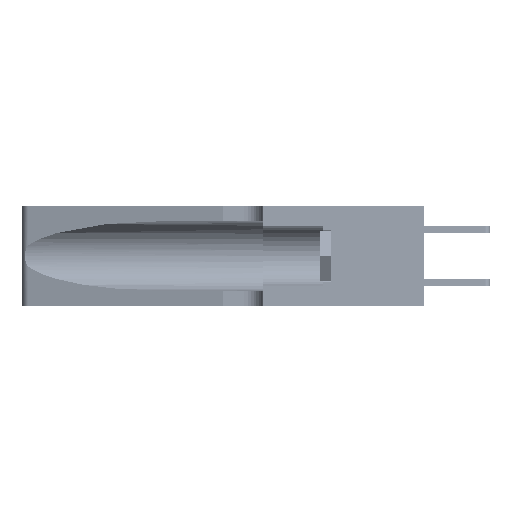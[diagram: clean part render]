
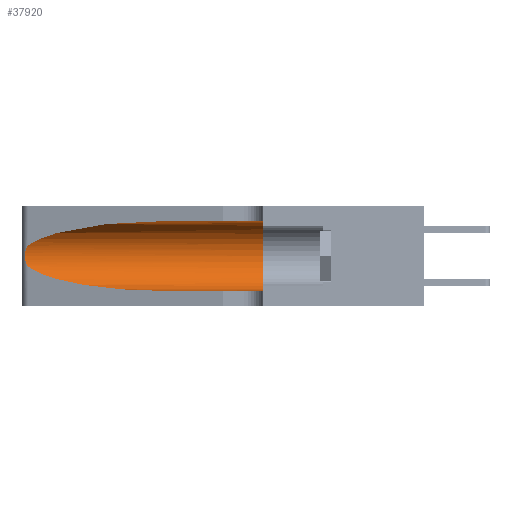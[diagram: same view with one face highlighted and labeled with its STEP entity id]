
A CAD part, left-side view. The second image highlights one B-rep face of the part: STEP entity #37920.
In plain terms, the highlighted cylindrical face has radius 3.308 mm (diameter 6.617 mm), a partial arc.
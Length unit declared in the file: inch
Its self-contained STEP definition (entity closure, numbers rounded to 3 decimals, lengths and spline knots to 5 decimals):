
#513 = CARTESIAN_POINT ( 'NONE',  ( 0.1305, 0.35, 0.185 ) ) ;
#750 = CIRCLE ( 'NONE', #49949, 0.13025 ) ;
#852 = VERTEX_POINT ( 'NONE', #14335 ) ;
#1556 =( BOUNDED_CURVE ( )  B_SPLINE_CURVE ( 3, ( #27196, #48484, #35395, #31410 ),
 .UNSPECIFIED., .F., .T. ) 
 B_SPLINE_CURVE_WITH_KNOTS ( ( 4, 4 ),
 ( 3.44316, 4.71239 ),
 .UNSPECIFIED. ) 
 CURVE ( )  GEOMETRIC_REPRESENTATION_ITEM ( )  RATIONAL_B_SPLINE_CURVE ( ( 1., 0.87, 0.87, 1. ) ) 
 REPRESENTATION_ITEM ( '' )  );
#1762 = CARTESIAN_POINT ( 'NONE',  ( 0.1305, 1.61858, 0.31525 ) ) ;
#3126 = CARTESIAN_POINT ( 'NONE',  ( 0.25555, 1.22994, 0.2215 ) ) ;
#3614 = ORIENTED_EDGE ( 'NONE', *, *, #16520, .F. ) ;
#4356 = DIRECTION ( 'NONE',  ( 0., 0., 1. ) ) ;
#5563 = CARTESIAN_POINT ( 'NONE',  ( 0.1305, 1.61858, 0.185 ) ) ;
#5946 = EDGE_LOOP ( 'NONE', ( #40991, #8715, #35002, #17758, #3614, #28600 ) ) ;
#7328 = CARTESIAN_POINT ( 'NONE',  ( 0.25856, 1.23593, 0.16098 ) ) ;
#8598 = VECTOR ( 'NONE', #21838, 39.37008 ) ;
#8715 = ORIENTED_EDGE ( 'NONE', *, *, #25585, .T. ) ;
#8809 = VERTEX_POINT ( 'NONE', #23151 ) ;
#9254 = DIRECTION ( 'NONE',  ( 0., 1., 0. ) ) ;
#10370 = EDGE_CURVE ( 'NONE', #8809, #38213, #12189, .T. ) ;
#10957 = CARTESIAN_POINT ( 'NONE',  ( 0.25487, 1.22718, 0.22369 ) ) ;
#11316 = CARTESIAN_POINT ( 'NONE',  ( 0.25555, 1.22993, 0.14849 ) ) ;
#12012 = CARTESIAN_POINT ( 'NONE',  ( 0.25487, 1.22718, 0.14631 ) ) ;
#12189 = LINE ( 'NONE', #1762, #20646 ) ;
#13992 = VERTEX_POINT ( 'NONE', #45386 ) ;
#14335 = CARTESIAN_POINT ( 'NONE',  ( 0.25487, 1.22718, 0.22369 ) ) ;
#14956 = CARTESIAN_POINT ( 'NONE',  ( 0.25639, 1.23186, 0.15144 ) ) ;
#15243 =( BOUNDED_CURVE ( )  B_SPLINE_CURVE ( 3, ( #47153, #22226, #26943, #43481 ),
 .UNSPECIFIED., .F., .F. ) 
 B_SPLINE_CURVE_WITH_KNOTS ( ( 4, 4 ),
 ( 1.5708, 2.84003 ),
 .UNSPECIFIED. ) 
 CURVE ( )  GEOMETRIC_REPRESENTATION_ITEM ( )  RATIONAL_B_SPLINE_CURVE ( ( 1., 0.87, 0.87, 1. ) ) 
 REPRESENTATION_ITEM ( '' )  );
#15687 = CARTESIAN_POINT ( 'NONE',  ( 0.25487, 1.22718, 0.14631 ) ) ;
#16520 = EDGE_CURVE ( 'NONE', #38213, #19927, #750, .T. ) ;
#17758 = ORIENTED_EDGE ( 'NONE', *, *, #53254, .T. ) ;
#18133 = VERTEX_POINT ( 'NONE', #12012 ) ;
#19146 = CARTESIAN_POINT ( 'NONE',  ( 0.25639, 1.23184, 0.21858 ) ) ;
#19323 = CARTESIAN_POINT ( 'NONE',  ( 0.26018, 1.23835, 0.19895 ) ) ;
#19927 = VERTEX_POINT ( 'NONE', #27743 ) ;
#20646 = VECTOR ( 'NONE', #52000, 39.37008 ) ;
#21592 = DIRECTION ( 'NONE',  ( 0., 0., -1. ) ) ;
#21838 = DIRECTION ( 'NONE',  ( 0., -1., 0. ) ) ;
#22226 = CARTESIAN_POINT ( 'NONE',  ( 0.18966, 0.96281, 0.31525 ) ) ;
#22706 = FACE_OUTER_BOUND ( 'NONE', #5946, .T. ) ;
#23151 = CARTESIAN_POINT ( 'NONE',  ( 0.1305, 0.72297, 0.31525 ) ) ;
#23886 = CARTESIAN_POINT ( 'NONE',  ( 0.26017, 1.23833, 0.17102 ) ) ;
#24083 = CARTESIAN_POINT ( 'NONE',  ( 0.26075, 1.23896, 0.178 ) ) ;
#25585 = EDGE_CURVE ( 'NONE', #852, #18133, #35574, .T. ) ;
#26383 = CARTESIAN_POINT ( 'NONE',  ( 0.1305, 1.61858, 0.05475 ) ) ;
#26943 = CARTESIAN_POINT ( 'NONE',  ( 0.2373, 1.15595, 0.28018 ) ) ;
#27196 = CARTESIAN_POINT ( 'NONE',  ( 0.25487, 1.22718, 0.14631 ) ) ;
#27743 = CARTESIAN_POINT ( 'NONE',  ( 0.1305, 0.35, 0.05475 ) ) ;
#28247 = CARTESIAN_POINT ( 'NONE',  ( 0.25854, 1.2359, 0.20912 ) ) ;
#28600 = ORIENTED_EDGE ( 'NONE', *, *, #10370, .F. ) ;
#31410 = CARTESIAN_POINT ( 'NONE',  ( 0.1305, 0.72297, 0.05475 ) ) ;
#31916 = CARTESIAN_POINT ( 'NONE',  ( 0.26075, 1.23896, 0.19203 ) ) ;
#33375 = EDGE_CURVE ( 'NONE', #8809, #852, #15243, .T. ) ;
#33853 = AXIS2_PLACEMENT_3D ( 'NONE', #5563, #33961, #21592 ) ;
#33961 = DIRECTION ( 'NONE',  ( 0., -1., 0. ) ) ;
#35002 = ORIENTED_EDGE ( 'NONE', *, *, #40027, .T. ) ;
#35395 = CARTESIAN_POINT ( 'NONE',  ( 0.18966, 0.96281, 0.05475 ) ) ;
#35574 = B_SPLINE_CURVE_WITH_KNOTS ( 'NONE', 3,
 ( #10957, #3126, #19146, #35889, #28247, #19323, #31916, #24083, #23886, #7328, #40620, #14956, #11316, #15687 ),
 .UNSPECIFIED., .F., .F.,
 ( 4, 2, 2, 2, 2, 2, 4 ),
 ( 0., 0.00027, 0.00053, 0.00107, 0.0016, 0.00187, 0.00214 ),
 .UNSPECIFIED. ) ;
#35889 = CARTESIAN_POINT ( 'NONE',  ( 0.25787, 1.23484, 0.2124 ) ) ;
#37920 = ADVANCED_FACE ( 'NONE', ( #22706 ), #48703, .F. ) ;
#38213 = VERTEX_POINT ( 'NONE', #44100 ) ;
#40027 = EDGE_CURVE ( 'NONE', #18133, #13992, #1556, .T. ) ;
#40620 = CARTESIAN_POINT ( 'NONE',  ( 0.25789, 1.23486, 0.15765 ) ) ;
#40991 = ORIENTED_EDGE ( 'NONE', *, *, #33375, .T. ) ;
#43481 = CARTESIAN_POINT ( 'NONE',  ( 0.25487, 1.22718, 0.22369 ) ) ;
#44100 = CARTESIAN_POINT ( 'NONE',  ( 0.1305, 0.35, 0.31525 ) ) ;
#45386 = CARTESIAN_POINT ( 'NONE',  ( 0.1305, 0.72297, 0.05475 ) ) ;
#47025 = LINE ( 'NONE', #26383, #8598 ) ;
#47153 = CARTESIAN_POINT ( 'NONE',  ( 0.1305, 0.72297, 0.31525 ) ) ;
#48484 = CARTESIAN_POINT ( 'NONE',  ( 0.2373, 1.15595, 0.08982 ) ) ;
#48703 = CYLINDRICAL_SURFACE ( 'NONE', #33853, 0.13025 ) ;
#49949 = AXIS2_PLACEMENT_3D ( 'NONE', #513, #9254, #4356 ) ;
#52000 = DIRECTION ( 'NONE',  ( 0., -1., 0. ) ) ;
#53254 = EDGE_CURVE ( 'NONE', #13992, #19927, #47025, .T. ) ;
